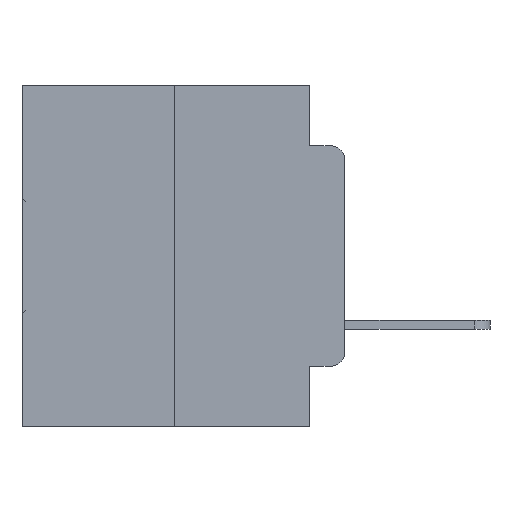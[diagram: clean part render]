
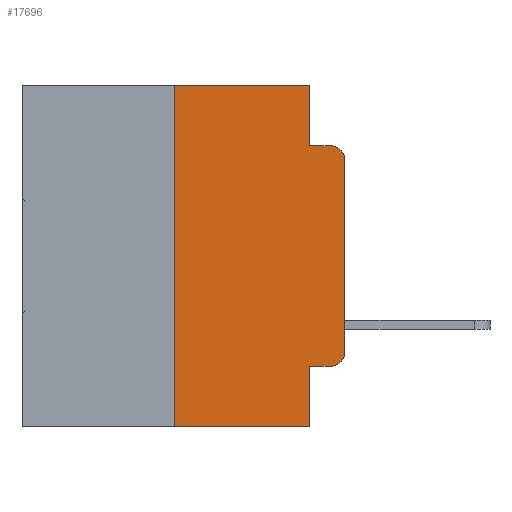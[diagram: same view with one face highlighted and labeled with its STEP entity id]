
A CAD part, left-side view. The second image highlights one B-rep face of the part: STEP entity #17696.
In plain terms, the highlighted planar face has unit normal (-1, 0, 0).
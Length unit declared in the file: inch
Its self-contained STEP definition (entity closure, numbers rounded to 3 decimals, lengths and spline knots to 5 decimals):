
#229 = VECTOR ( 'NONE', #1507, 39.37008 ) ;
#232 = CARTESIAN_POINT ( 'NONE',  ( 0., 0., -0.1085 ) ) ;
#586 = EDGE_CURVE ( 'NONE', #12310, #15966, #31229, .T. ) ;
#1274 = LINE ( 'NONE', #20063, #20506 ) ;
#1507 = DIRECTION ( 'NONE',  ( 0., -1., 0. ) ) ;
#2270 = ORIENTED_EDGE ( 'NONE', *, *, #3816, .F. ) ;
#2528 = DIRECTION ( 'NONE',  ( 0., 0., -1. ) ) ;
#3023 = CARTESIAN_POINT ( 'NONE',  ( 0., 0.051, -0.0885 ) ) ;
#3250 = CARTESIAN_POINT ( 'NONE',  ( 0., 0.051, -0.4115 ) ) ;
#3599 = CARTESIAN_POINT ( 'NONE',  ( 0., 0.02, -0.3915 ) ) ;
#3816 = EDGE_CURVE ( 'NONE', #24700, #12300, #19300, .T. ) ;
#4349 = ORIENTED_EDGE ( 'NONE', *, *, #23369, .T. ) ;
#5277 = CARTESIAN_POINT ( 'NONE',  ( 0., 0.051, -0.0885 ) ) ;
#5949 = DIRECTION ( 'NONE',  ( 0., -1., 0. ) ) ;
#6042 = ORIENTED_EDGE ( 'NONE', *, *, #10891, .F. ) ;
#6259 = DIRECTION ( 'NONE',  ( 0., 0., -1. ) ) ;
#6808 = DIRECTION ( 'NONE',  ( 0., 0., 1. ) ) ;
#7287 = LINE ( 'NONE', #19031, #229 ) ;
#7634 = CARTESIAN_POINT ( 'NONE',  ( 0., 0.473, 0. ) ) ;
#7689 = VERTEX_POINT ( 'NONE', #26156 ) ;
#8141 = CARTESIAN_POINT ( 'NONE',  ( 0., 0.473, -0.5 ) ) ;
#8296 = CARTESIAN_POINT ( 'NONE',  ( 0., 0.25, -0.5 ) ) ;
#8920 = LINE ( 'NONE', #27742, #21140 ) ;
#9360 = EDGE_CURVE ( 'NONE', #22558, #12300, #17062, .T. ) ;
#9641 = LINE ( 'NONE', #21056, #21121 ) ;
#10690 = DIRECTION ( 'NONE',  ( 0., -1., 0. ) ) ;
#10891 = EDGE_CURVE ( 'NONE', #15966, #30475, #22670, .T. ) ;
#10951 = EDGE_CURVE ( 'NONE', #24700, #16681, #8920, .T. ) ;
#11781 = VERTEX_POINT ( 'NONE', #20220 ) ;
#12300 = VERTEX_POINT ( 'NONE', #12795 ) ;
#12310 = VERTEX_POINT ( 'NONE', #22530 ) ;
#12546 = DIRECTION ( 'NONE',  ( 0., 0., -1. ) ) ;
#12596 = ORIENTED_EDGE ( 'NONE', *, *, #586, .F. ) ;
#12738 = EDGE_CURVE ( 'NONE', #11781, #12310, #7287, .T. ) ;
#12795 = CARTESIAN_POINT ( 'NONE',  ( 0., 0.051, -0.5 ) ) ;
#12949 = CARTESIAN_POINT ( 'NONE',  ( 0., 0.051, 0. ) ) ;
#13162 = CARTESIAN_POINT ( 'NONE',  ( 0., 0.02, -0.4115 ) ) ;
#13190 = CARTESIAN_POINT ( 'NONE',  ( 0., 0.02, -0.0885 ) ) ;
#14169 = ORIENTED_EDGE ( 'NONE', *, *, #19183, .F. ) ;
#14228 = AXIS2_PLACEMENT_3D ( 'NONE', #7634, #26985, #12546 ) ;
#15966 = VERTEX_POINT ( 'NONE', #5277 ) ;
#16216 = VECTOR ( 'NONE', #10690, 39.37008 ) ;
#16248 = DIRECTION ( 'NONE',  ( 0., 0., -1. ) ) ;
#16500 = ORIENTED_EDGE ( 'NONE', *, *, #10951, .T. ) ;
#16681 = VERTEX_POINT ( 'NONE', #13162 ) ;
#17062 = LINE ( 'NONE', #8141, #22762 ) ;
#17582 = DIRECTION ( 'NONE',  ( -1., 0., 0. ) ) ;
#17696 = ADVANCED_FACE ( 'NONE', ( #24795 ), #22257, .F. ) ;
#19031 = CARTESIAN_POINT ( 'NONE',  ( 0., 0.473, 0. ) ) ;
#19183 = EDGE_CURVE ( 'NONE', #22558, #11781, #1274, .T. ) ;
#19300 = LINE ( 'NONE', #12949, #30099 ) ;
#19757 = CIRCLE ( 'NONE', #29501, 0.02 ) ;
#19817 = EDGE_CURVE ( 'NONE', #16681, #7689, #19757, .T. ) ;
#19893 = ORIENTED_EDGE ( 'NONE', *, *, #12738, .F. ) ;
#20063 = CARTESIAN_POINT ( 'NONE',  ( 0., 0.25, 0. ) ) ;
#20220 = CARTESIAN_POINT ( 'NONE',  ( 0., 0.25, 0. ) ) ;
#20506 = VECTOR ( 'NONE', #22505, 39.37008 ) ;
#20640 = ORIENTED_EDGE ( 'NONE', *, *, #9360, .T. ) ;
#20953 = DIRECTION ( 'NONE',  ( -1., 0., 0. ) ) ;
#21056 = CARTESIAN_POINT ( 'NONE',  ( 0., 0., 0. ) ) ;
#21121 = VECTOR ( 'NONE', #6808, 39.37008 ) ;
#21140 = VECTOR ( 'NONE', #5949, 39.37008 ) ;
#21648 = EDGE_CURVE ( 'NONE', #7689, #22501, #9641, .T. ) ;
#22102 = CIRCLE ( 'NONE', #25910, 0.02 ) ;
#22257 = PLANE ( 'NONE',  #14228 ) ;
#22501 = VERTEX_POINT ( 'NONE', #232 ) ;
#22505 = DIRECTION ( 'NONE',  ( 0., 0., 1. ) ) ;
#22530 = CARTESIAN_POINT ( 'NONE',  ( 0., 0.051, 0. ) ) ;
#22558 = VERTEX_POINT ( 'NONE', #8296 ) ;
#22670 = LINE ( 'NONE', #3023, #16216 ) ;
#22762 = VECTOR ( 'NONE', #29598, 39.37008 ) ;
#23369 = EDGE_CURVE ( 'NONE', #22501, #30475, #22102, .T. ) ;
#24700 = VERTEX_POINT ( 'NONE', #3250 ) ;
#24795 = FACE_OUTER_BOUND ( 'NONE', #27002, .T. ) ;
#25491 = VECTOR ( 'NONE', #16248, 39.37008 ) ;
#25910 = AXIS2_PLACEMENT_3D ( 'NONE', #31330, #17582, #2528 ) ;
#26156 = CARTESIAN_POINT ( 'NONE',  ( 0., 0., -0.3915 ) ) ;
#26985 = DIRECTION ( 'NONE',  ( 1., 0., 0. ) ) ;
#27002 = EDGE_LOOP ( 'NONE', ( #29301, #4349, #6042, #12596, #19893, #14169, #20640, #2270, #16500, #28965 ) ) ;
#27742 = CARTESIAN_POINT ( 'NONE',  ( 0., 0.051, -0.4115 ) ) ;
#28155 = DIRECTION ( 'NONE',  ( 0., 0., -1. ) ) ;
#28934 = CARTESIAN_POINT ( 'NONE',  ( 0., 0.051, 0. ) ) ;
#28965 = ORIENTED_EDGE ( 'NONE', *, *, #19817, .T. ) ;
#29301 = ORIENTED_EDGE ( 'NONE', *, *, #21648, .T. ) ;
#29501 = AXIS2_PLACEMENT_3D ( 'NONE', #3599, #20953, #6259 ) ;
#29598 = DIRECTION ( 'NONE',  ( 0., -1., 0. ) ) ;
#30099 = VECTOR ( 'NONE', #28155, 39.37008 ) ;
#30475 = VERTEX_POINT ( 'NONE', #13190 ) ;
#31229 = LINE ( 'NONE', #28934, #25491 ) ;
#31330 = CARTESIAN_POINT ( 'NONE',  ( 0., 0.02, -0.1085 ) ) ;
